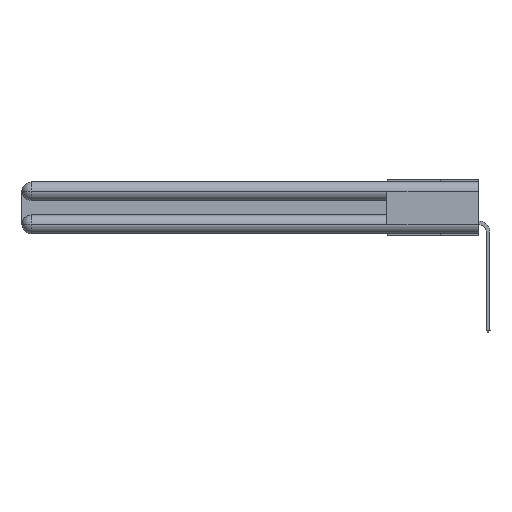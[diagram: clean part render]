
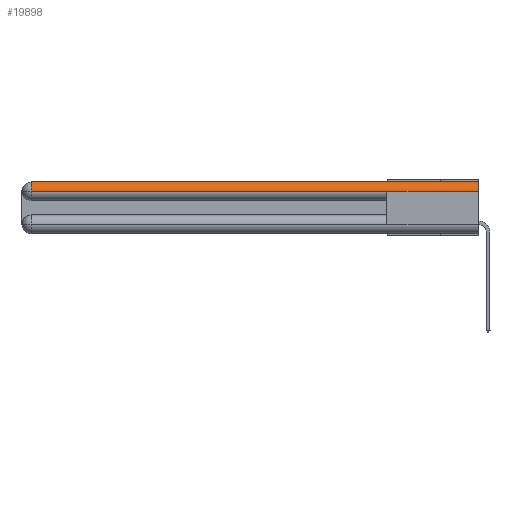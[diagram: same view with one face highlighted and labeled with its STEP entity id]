
A CAD part, left-side view. The second image highlights one B-rep face of the part: STEP entity #19898.
In plain terms, the highlighted cylindrical face has radius 1.562 mm (diameter 3.124 mm), a partial arc.
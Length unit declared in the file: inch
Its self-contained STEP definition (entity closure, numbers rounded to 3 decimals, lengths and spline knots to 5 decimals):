
#318 = EDGE_CURVE ( 'NONE', #3319, #13831, #15452, .T. ) ;
#1045 = EDGE_CURVE ( 'NONE', #15056, #3319, #25451, .T. ) ;
#1914 = EDGE_CURVE ( 'NONE', #13831, #17096, #18509, .T. ) ;
#2469 = DIRECTION ( 'NONE',  ( 0., 1., 0. ) ) ;
#2635 = CYLINDRICAL_SURFACE ( 'NONE', #9143, 0.0615 ) ;
#3319 = VERTEX_POINT ( 'NONE', #26173 ) ;
#3555 = CARTESIAN_POINT ( 'NONE',  ( 0.0615, 0., 0. ) ) ;
#3701 = DIRECTION ( 'NONE',  ( 0., -1., 0. ) ) ;
#3913 = DIRECTION ( 'NONE',  ( 0., 1., 0. ) ) ;
#4227 = VECTOR ( 'NONE', #2469, 39.37008 ) ;
#4648 = DIRECTION ( 'NONE',  ( 0., -1., 0. ) ) ;
#4729 = CARTESIAN_POINT ( 'NONE',  ( 0.0615, 0., -0.0615 ) ) ;
#5472 = AXIS2_PLACEMENT_3D ( 'NONE', #4729, #4648, #22342 ) ;
#6005 = ORIENTED_EDGE ( 'NONE', *, *, #18212, .T. ) ;
#6192 = CARTESIAN_POINT ( 'NONE',  ( 0.0615, 0., -0.0615 ) ) ;
#6950 = EDGE_LOOP ( 'NONE', ( #29010, #11241, #6005, #27855, #18578 ) ) ;
#7099 = DIRECTION ( 'NONE',  ( 0., 0., 1. ) ) ;
#9143 = AXIS2_PLACEMENT_3D ( 'NONE', #6192, #3913, #10992 ) ;
#10314 = CARTESIAN_POINT ( 'NONE',  ( 0., 3., -0.0615 ) ) ;
#10992 = DIRECTION ( 'NONE',  ( 0., 0., 1. ) ) ;
#11241 = ORIENTED_EDGE ( 'NONE', *, *, #14787, .T. ) ;
#12774 = VECTOR ( 'NONE', #3701, 39.37008 ) ;
#13831 = VERTEX_POINT ( 'NONE', #26248 ) ;
#13912 = DIRECTION ( 'NONE',  ( 0., -1., 0. ) ) ;
#13994 = CARTESIAN_POINT ( 'NONE',  ( 0.0615, 2.94, -0.0615 ) ) ;
#14217 = CARTESIAN_POINT ( 'NONE',  ( 0., 0.6, -0.0615 ) ) ;
#14787 = EDGE_CURVE ( 'NONE', #15056, #26245, #17643, .T. ) ;
#14795 = FACE_OUTER_BOUND ( 'NONE', #6950, .T. ) ;
#15056 = VERTEX_POINT ( 'NONE', #26401 ) ;
#15452 = CIRCLE ( 'NONE', #5472, 0.0615 ) ;
#17056 = LINE ( 'NONE', #10314, #12774 ) ;
#17096 = VERTEX_POINT ( 'NONE', #14217 ) ;
#17643 = CIRCLE ( 'NONE', #28011, 0.0615 ) ;
#18212 = EDGE_CURVE ( 'NONE', #26245, #17096, #17056, .T. ) ;
#18509 = LINE ( 'NONE', #20828, #4227 ) ;
#18578 = ORIENTED_EDGE ( 'NONE', *, *, #318, .F. ) ;
#18823 = CARTESIAN_POINT ( 'NONE',  ( 0., 2.94, -0.0615 ) ) ;
#19898 = ADVANCED_FACE ( 'NONE', ( #14795 ), #2635, .T. ) ;
#20828 = CARTESIAN_POINT ( 'NONE',  ( 0., 3., -0.0615 ) ) ;
#22342 = DIRECTION ( 'NONE',  ( 1., 0., 0. ) ) ;
#25451 = LINE ( 'NONE', #3555, #28693 ) ;
#26173 = CARTESIAN_POINT ( 'NONE',  ( 0.0615, 0., 0. ) ) ;
#26245 = VERTEX_POINT ( 'NONE', #18823 ) ;
#26248 = CARTESIAN_POINT ( 'NONE',  ( 0., 0., -0.0615 ) ) ;
#26401 = CARTESIAN_POINT ( 'NONE',  ( 0.0615, 2.94, 0. ) ) ;
#26535 = DIRECTION ( 'NONE',  ( 0., -1., 0. ) ) ;
#27855 = ORIENTED_EDGE ( 'NONE', *, *, #1914, .F. ) ;
#28011 = AXIS2_PLACEMENT_3D ( 'NONE', #13994, #13912, #7099 ) ;
#28693 = VECTOR ( 'NONE', #26535, 39.37008 ) ;
#29010 = ORIENTED_EDGE ( 'NONE', *, *, #1045, .F. ) ;
